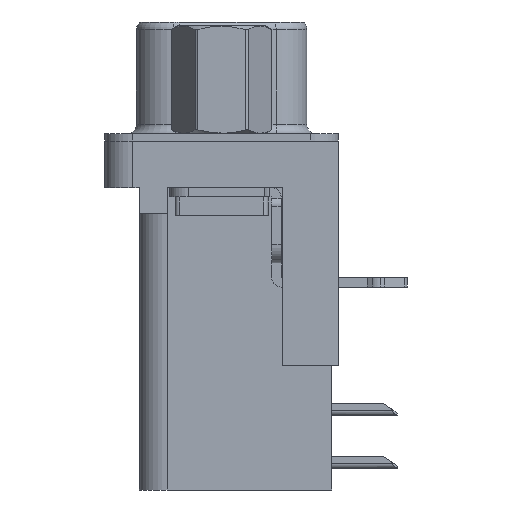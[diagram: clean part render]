
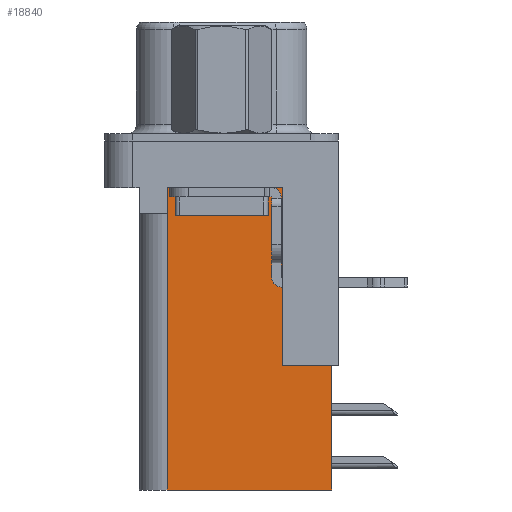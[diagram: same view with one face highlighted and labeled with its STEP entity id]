
A CAD part, left-side view. The second image highlights one B-rep face of the part: STEP entity #18840.
In plain terms, the highlighted planar face has unit normal (-1, 0, 0).
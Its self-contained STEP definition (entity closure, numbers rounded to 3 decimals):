
#89 = EDGE_CURVE ( 'NONE', #15357, #18115, #19436, .T. ) ;
#339 = VERTEX_POINT ( 'NONE', #23305 ) ;
#359 = CARTESIAN_POINT ( 'NONE',  ( 3.765, -3.295, -18.76 ) ) ;
#457 = VECTOR ( 'NONE', #22730, 1000. ) ;
#1134 = ORIENTED_EDGE ( 'NONE', *, *, #14000, .F. ) ;
#1751 = VECTOR ( 'NONE', #7621, 1000. ) ;
#1808 = VERTEX_POINT ( 'NONE', #18807 ) ;
#1956 = CARTESIAN_POINT ( 'NONE',  ( 3.765, -6.295, -12.05 ) ) ;
#2085 = CARTESIAN_POINT ( 'NONE',  ( 3.765, -3.295, -12.05 ) ) ;
#2373 = DIRECTION ( 'NONE',  ( 0., 1., 0. ) ) ;
#3034 = LINE ( 'NONE', #21231, #22615 ) ;
#4110 = PLANE ( 'NONE',  #18813 ) ;
#4434 = VECTOR ( 'NONE', #16389, 1000. ) ;
#4568 = VERTEX_POINT ( 'NONE', #14957 ) ;
#5185 = ORIENTED_EDGE ( 'NONE', *, *, #12707, .T. ) ;
#5808 = EDGE_LOOP ( 'NONE', ( #15207, #5185, #12888, #1134, #21588, #20163, #8800, #12202 ) ) ;
#6022 = DIRECTION ( 'NONE',  ( 1., 0., 0. ) ) ;
#6410 = CARTESIAN_POINT ( 'NONE',  ( 3.765, -3.295, -2.5 ) ) ;
#6630 = VERTEX_POINT ( 'NONE', #17462 ) ;
#6709 = LINE ( 'NONE', #19006, #1751 ) ;
#6890 = LINE ( 'NONE', #24251, #10604 ) ;
#7621 = DIRECTION ( 'NONE',  ( 0., 0., 1. ) ) ;
#8107 = LINE ( 'NONE', #11524, #17646 ) ;
#8800 = ORIENTED_EDGE ( 'NONE', *, *, #13173, .T. ) ;
#9940 = CARTESIAN_POINT ( 'NONE',  ( 3.765, -3.295, -18.76 ) ) ;
#10454 = LINE ( 'NONE', #1956, #457 ) ;
#10604 = VECTOR ( 'NONE', #12883, 1000. ) ;
#11361 = VECTOR ( 'NONE', #2373, 1000. ) ;
#11524 = CARTESIAN_POINT ( 'NONE',  ( 3.765, 2.895, -3.9 ) ) ;
#12202 = ORIENTED_EDGE ( 'NONE', *, *, #23647, .T. ) ;
#12707 = EDGE_CURVE ( 'NONE', #1808, #15357, #8107, .T. ) ;
#12824 = EDGE_CURVE ( 'NONE', #6630, #4568, #15818, .T. ) ;
#12883 = DIRECTION ( 'NONE',  ( 0., 1., 0. ) ) ;
#12888 = ORIENTED_EDGE ( 'NONE', *, *, #89, .T. ) ;
#13173 = EDGE_CURVE ( 'NONE', #339, #16970, #10454, .T. ) ;
#13177 = DIRECTION ( 'NONE',  ( 0., 1., 0. ) ) ;
#13456 = DIRECTION ( 'NONE',  ( 0., 0., -1. ) ) ;
#14000 = EDGE_CURVE ( 'NONE', #4568, #18115, #3034, .T. ) ;
#14957 = CARTESIAN_POINT ( 'NONE',  ( 3.765, 2.925, -18.76 ) ) ;
#15207 = ORIENTED_EDGE ( 'NONE', *, *, #19314, .T. ) ;
#15357 = VERTEX_POINT ( 'NONE', #21421 ) ;
#15818 = LINE ( 'NONE', #9940, #11361 ) ;
#16389 = DIRECTION ( 'NONE',  ( 0., 0., -1. ) ) ;
#16645 = EDGE_CURVE ( 'NONE', #339, #6630, #20790, .T. ) ;
#16970 = VERTEX_POINT ( 'NONE', #2085 ) ;
#17462 = CARTESIAN_POINT ( 'NONE',  ( 3.765, -5.925, -18.76 ) ) ;
#17646 = VECTOR ( 'NONE', #13456, 1000. ) ;
#18115 = VERTEX_POINT ( 'NONE', #22333 ) ;
#18807 = CARTESIAN_POINT ( 'NONE',  ( 3.765, 2.895, -2.5 ) ) ;
#18813 = AXIS2_PLACEMENT_3D ( 'NONE', #359, #6022, #19303 ) ;
#18840 = ADVANCED_FACE ( 'NONE', ( #19576 ), #4110, .F. ) ;
#19006 = CARTESIAN_POINT ( 'NONE',  ( 3.765, -3.295, -18.76 ) ) ;
#19044 = VERTEX_POINT ( 'NONE', #6410 ) ;
#19303 = DIRECTION ( 'NONE',  ( 0., 1., 0. ) ) ;
#19314 = EDGE_CURVE ( 'NONE', #19044, #1808, #6890, .T. ) ;
#19436 = LINE ( 'NONE', #21627, #23877 ) ;
#19576 = FACE_OUTER_BOUND ( 'NONE', #5808, .T. ) ;
#20163 = ORIENTED_EDGE ( 'NONE', *, *, #16645, .F. ) ;
#20790 = LINE ( 'NONE', #22039, #4434 ) ;
#21231 = CARTESIAN_POINT ( 'NONE',  ( 3.765, 2.925, -18.76 ) ) ;
#21421 = CARTESIAN_POINT ( 'NONE',  ( 3.765, 2.895, -3.9 ) ) ;
#21588 = ORIENTED_EDGE ( 'NONE', *, *, #12824, .F. ) ;
#21627 = CARTESIAN_POINT ( 'NONE',  ( 3.765, 0., -3.9 ) ) ;
#22039 = CARTESIAN_POINT ( 'NONE',  ( 3.765, -5.925, -2. ) ) ;
#22333 = CARTESIAN_POINT ( 'NONE',  ( 3.765, 2.925, -3.9 ) ) ;
#22615 = VECTOR ( 'NONE', #23154, 1000. ) ;
#22730 = DIRECTION ( 'NONE',  ( 0., 1., 0. ) ) ;
#23154 = DIRECTION ( 'NONE',  ( 0., 0., 1. ) ) ;
#23305 = CARTESIAN_POINT ( 'NONE',  ( 3.765, -5.925, -12.05 ) ) ;
#23647 = EDGE_CURVE ( 'NONE', #16970, #19044, #6709, .T. ) ;
#23877 = VECTOR ( 'NONE', #13177, 1000. ) ;
#24251 = CARTESIAN_POINT ( 'NONE',  ( 3.765, -3.295, -2.5 ) ) ;
